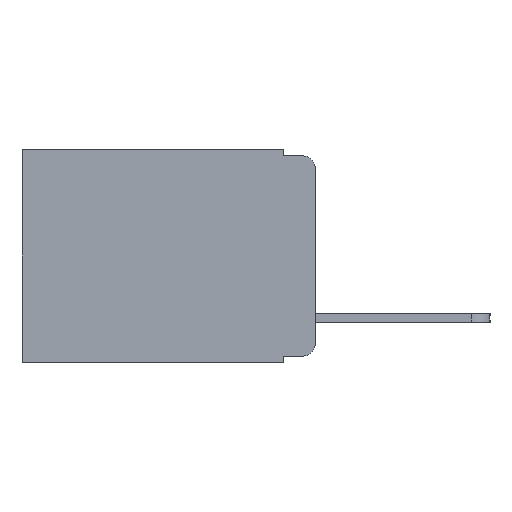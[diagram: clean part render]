
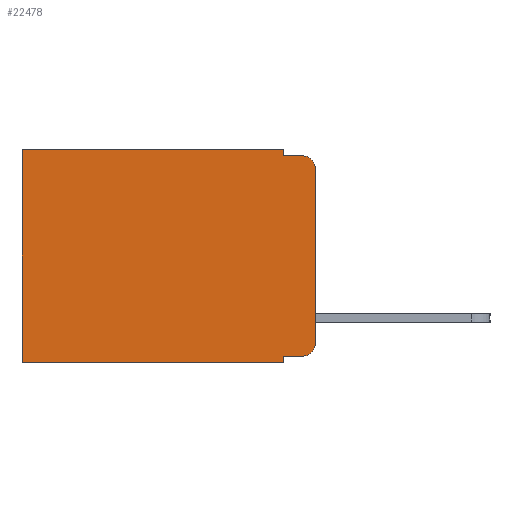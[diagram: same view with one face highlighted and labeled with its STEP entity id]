
A CAD part, left-side view. The second image highlights one B-rep face of the part: STEP entity #22478.
In plain terms, the highlighted planar face has unit normal (-1, 0, 0).
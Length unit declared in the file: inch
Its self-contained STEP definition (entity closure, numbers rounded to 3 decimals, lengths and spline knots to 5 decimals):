
#102 = DIRECTION ( 'NONE',  ( -1., 0., 0. ) ) ;
#232 = VERTEX_POINT ( 'NONE', #4737 ) ;
#427 = DIRECTION ( 'NONE',  ( 0., 0., -1. ) ) ;
#858 = VECTOR ( 'NONE', #12671, 39.37008 ) ;
#1328 = VERTEX_POINT ( 'NONE', #15012 ) ;
#1891 = EDGE_CURVE ( 'NONE', #1328, #18239, #4590, .T. ) ;
#2016 = DIRECTION ( 'NONE',  ( 0., 0., -1. ) ) ;
#2408 = VERTEX_POINT ( 'NONE', #9540 ) ;
#3250 = DIRECTION ( 'NONE',  ( 0., 0., -1. ) ) ;
#3416 = DIRECTION ( 'NONE',  ( -1., 0., 0. ) ) ;
#4044 = EDGE_CURVE ( 'NONE', #13977, #2408, #22786, .T. ) ;
#4059 = ORIENTED_EDGE ( 'NONE', *, *, #1891, .T. ) ;
#4293 = CARTESIAN_POINT ( 'NONE',  ( 0.298, 0., -0.03 ) ) ;
#4365 = LINE ( 'NONE', #13133, #18508 ) ;
#4433 = CARTESIAN_POINT ( 'NONE',  ( 0.298, 0.051, -0.333 ) ) ;
#4590 = LINE ( 'NONE', #13735, #21786 ) ;
#4737 = CARTESIAN_POINT ( 'NONE',  ( 0.298, 0.051, -0.343 ) ) ;
#4780 = EDGE_CURVE ( 'NONE', #10707, #4886, #11711, .T. ) ;
#4886 = VERTEX_POINT ( 'NONE', #5667 ) ;
#5108 = EDGE_LOOP ( 'NONE', ( #15765, #10265, #20085, #22505, #11557, #4059, #22861, #19763, #23356, #22620 ) ) ;
#5268 = LINE ( 'NONE', #16248, #9633 ) ;
#5390 = DIRECTION ( 'NONE',  ( 0., 1., 0. ) ) ;
#5667 = CARTESIAN_POINT ( 'NONE',  ( 0.298, 0.02, -0.01 ) ) ;
#5797 = CARTESIAN_POINT ( 'NONE',  ( 0.298, 0.02, -0.03 ) ) ;
#6159 = VECTOR ( 'NONE', #9000, 39.37008 ) ;
#6205 = FACE_OUTER_BOUND ( 'NONE', #5108, .T. ) ;
#7082 = CARTESIAN_POINT ( 'NONE',  ( 0.298, 0., -0.343 ) ) ;
#7536 = CARTESIAN_POINT ( 'NONE',  ( 0.298, 0.051, -0.01 ) ) ;
#7668 = VECTOR ( 'NONE', #23335, 39.37008 ) ;
#7730 = DIRECTION ( 'NONE',  ( 1., 0., 0. ) ) ;
#8254 = VECTOR ( 'NONE', #5390, 39.37008 ) ;
#8317 = EDGE_CURVE ( 'NONE', #10528, #4886, #12587, .T. ) ;
#8841 = VERTEX_POINT ( 'NONE', #4433 ) ;
#9000 = DIRECTION ( 'NONE',  ( 0., -1., 0. ) ) ;
#9172 = EDGE_CURVE ( 'NONE', #8841, #232, #4365, .T. ) ;
#9540 = CARTESIAN_POINT ( 'NONE',  ( 0.298, 0., -0.313 ) ) ;
#9633 = VECTOR ( 'NONE', #3250, 39.37008 ) ;
#10265 = ORIENTED_EDGE ( 'NONE', *, *, #4780, .T. ) ;
#10528 = VERTEX_POINT ( 'NONE', #7536 ) ;
#10707 = VERTEX_POINT ( 'NONE', #4293 ) ;
#10739 = LINE ( 'NONE', #7082, #858 ) ;
#10863 = CARTESIAN_POINT ( 'NONE',  ( 0.298, 0.02, -0.333 ) ) ;
#11335 = CARTESIAN_POINT ( 'NONE',  ( 0.298, 0., 0. ) ) ;
#11557 = ORIENTED_EDGE ( 'NONE', *, *, #17173, .T. ) ;
#11631 = CARTESIAN_POINT ( 'NONE',  ( 0.298, 0.051, 0. ) ) ;
#11711 = CIRCLE ( 'NONE', #18622, 0.02 ) ;
#12219 = AXIS2_PLACEMENT_3D ( 'NONE', #23095, #102, #21376 ) ;
#12587 = LINE ( 'NONE', #23292, #7668 ) ;
#12671 = DIRECTION ( 'NONE',  ( 0., 1., 0. ) ) ;
#13133 = CARTESIAN_POINT ( 'NONE',  ( 0.298, 0.051, 0. ) ) ;
#13180 = LINE ( 'NONE', #18262, #8254 ) ;
#13223 = CARTESIAN_POINT ( 'NONE',  ( 0.298, 0.051, 0. ) ) ;
#13578 = LINE ( 'NONE', #13223, #17823 ) ;
#13735 = CARTESIAN_POINT ( 'NONE',  ( 0.298, 0.473, 0. ) ) ;
#13977 = VERTEX_POINT ( 'NONE', #10863 ) ;
#15012 = CARTESIAN_POINT ( 'NONE',  ( 0.298, 0.473, 0. ) ) ;
#15765 = ORIENTED_EDGE ( 'NONE', *, *, #23600, .F. ) ;
#16248 = CARTESIAN_POINT ( 'NONE',  ( 0.298, 0., 0. ) ) ;
#16555 = LINE ( 'NONE', #23437, #6159 ) ;
#17173 = EDGE_CURVE ( 'NONE', #23182, #1328, #13180, .T. ) ;
#17244 = CARTESIAN_POINT ( 'NONE',  ( 0.298, 0.473, -0.343 ) ) ;
#17350 = AXIS2_PLACEMENT_3D ( 'NONE', #11335, #7730, #20473 ) ;
#17538 = DIRECTION ( 'NONE',  ( 0., 0., -1. ) ) ;
#17823 = VECTOR ( 'NONE', #2016, 39.37008 ) ;
#17912 = EDGE_CURVE ( 'NONE', #8841, #13977, #16555, .T. ) ;
#18239 = VERTEX_POINT ( 'NONE', #17244 ) ;
#18262 = CARTESIAN_POINT ( 'NONE',  ( 0.298, 0., 0. ) ) ;
#18508 = VECTOR ( 'NONE', #17538, 39.37008 ) ;
#18622 = AXIS2_PLACEMENT_3D ( 'NONE', #5797, #3416, #19077 ) ;
#18670 = PLANE ( 'NONE',  #17350 ) ;
#19077 = DIRECTION ( 'NONE',  ( 0., 0., -1. ) ) ;
#19113 = EDGE_CURVE ( 'NONE', #232, #18239, #10739, .T. ) ;
#19763 = ORIENTED_EDGE ( 'NONE', *, *, #9172, .F. ) ;
#20085 = ORIENTED_EDGE ( 'NONE', *, *, #8317, .F. ) ;
#20473 = DIRECTION ( 'NONE',  ( 0., 0., -1. ) ) ;
#20693 = EDGE_CURVE ( 'NONE', #23182, #10528, #13578, .T. ) ;
#21376 = DIRECTION ( 'NONE',  ( 0., 0., -1. ) ) ;
#21786 = VECTOR ( 'NONE', #427, 39.37008 ) ;
#22478 = ADVANCED_FACE ( 'NONE', ( #6205 ), #18670, .F. ) ;
#22505 = ORIENTED_EDGE ( 'NONE', *, *, #20693, .F. ) ;
#22620 = ORIENTED_EDGE ( 'NONE', *, *, #4044, .T. ) ;
#22786 = CIRCLE ( 'NONE', #12219, 0.02 ) ;
#22861 = ORIENTED_EDGE ( 'NONE', *, *, #19113, .F. ) ;
#23095 = CARTESIAN_POINT ( 'NONE',  ( 0.298, 0.02, -0.313 ) ) ;
#23182 = VERTEX_POINT ( 'NONE', #11631 ) ;
#23292 = CARTESIAN_POINT ( 'NONE',  ( 0.298, 0.051, -0.01 ) ) ;
#23335 = DIRECTION ( 'NONE',  ( 0., -1., 0. ) ) ;
#23356 = ORIENTED_EDGE ( 'NONE', *, *, #17912, .T. ) ;
#23437 = CARTESIAN_POINT ( 'NONE',  ( 0.298, 0.051, -0.333 ) ) ;
#23600 = EDGE_CURVE ( 'NONE', #10707, #2408, #5268, .T. ) ;
